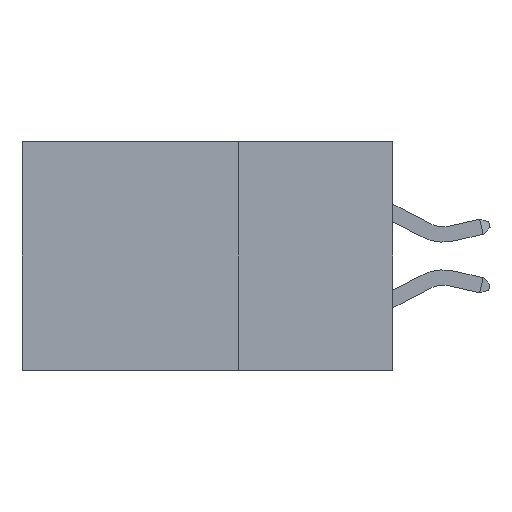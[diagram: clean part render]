
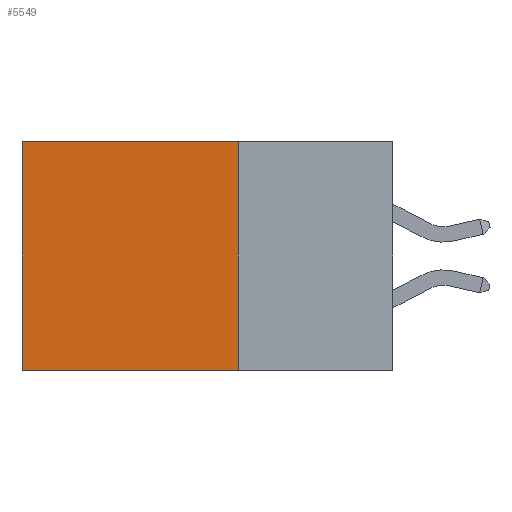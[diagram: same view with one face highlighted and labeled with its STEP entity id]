
A CAD part, left-side view. The second image highlights one B-rep face of the part: STEP entity #5549.
In plain terms, the highlighted planar face has unit normal (-1, 0, 0).
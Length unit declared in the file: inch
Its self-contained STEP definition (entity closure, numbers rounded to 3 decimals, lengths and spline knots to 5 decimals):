
#68 = VERTEX_POINT ( 'NONE', #19197 ) ;
#89 = DIRECTION ( 'NONE',  ( 1., 0., 0. ) ) ;
#135 = CARTESIAN_POINT ( 'NONE',  ( 0.2875, 0.25, 0. ) ) ;
#137 = CARTESIAN_POINT ( 'NONE',  ( 0.2875, 0.6, -0.37 ) ) ;
#147 = ORIENTED_EDGE ( 'NONE', *, *, #17305, .T. ) ;
#314 = DIRECTION ( 'NONE',  ( 0., 0., -1. ) ) ;
#1629 = DIRECTION ( 'NONE',  ( 0., 0., -1. ) ) ;
#2861 = ORIENTED_EDGE ( 'NONE', *, *, #16592, .F. ) ;
#3113 = VERTEX_POINT ( 'NONE', #137 ) ;
#3219 = DIRECTION ( 'NONE',  ( 0., 0., -1. ) ) ;
#3332 = CARTESIAN_POINT ( 'NONE',  ( 0.2875, 0.6, 0. ) ) ;
#3769 = CARTESIAN_POINT ( 'NONE',  ( 0.2875, 0.25, -0.37 ) ) ;
#3929 = PLANE ( 'NONE',  #12392 ) ;
#4336 = VECTOR ( 'NONE', #1629, 39.37008 ) ;
#5140 = DIRECTION ( 'NONE',  ( 0., 1., 0. ) ) ;
#5549 = ADVANCED_FACE ( 'NONE', ( #10672 ), #3929, .F. ) ;
#6506 = VECTOR ( 'NONE', #5140, 39.37008 ) ;
#6512 = VECTOR ( 'NONE', #6896, 39.37008 ) ;
#6896 = DIRECTION ( 'NONE',  ( 0., 1., 0. ) ) ;
#8709 = VECTOR ( 'NONE', #3219, 39.37008 ) ;
#9147 = CARTESIAN_POINT ( 'NONE',  ( 0.2875, 0.25, 0. ) ) ;
#9589 = EDGE_CURVE ( 'NONE', #68, #3113, #10535, .T. ) ;
#9916 = VERTEX_POINT ( 'NONE', #9147 ) ;
#10535 = LINE ( 'NONE', #3769, #6512 ) ;
#10672 = FACE_OUTER_BOUND ( 'NONE', #18408, .T. ) ;
#12073 = CARTESIAN_POINT ( 'NONE',  ( 0.2875, 0.6, 0. ) ) ;
#12135 = ORIENTED_EDGE ( 'NONE', *, *, #17420, .T. ) ;
#12392 = AXIS2_PLACEMENT_3D ( 'NONE', #135, #89, #314 ) ;
#13753 = CARTESIAN_POINT ( 'NONE',  ( 0.2875, 0.25, 0. ) ) ;
#14329 = LINE ( 'NONE', #15424, #6506 ) ;
#15424 = CARTESIAN_POINT ( 'NONE',  ( 0.2875, 0.25, 0. ) ) ;
#15942 = ORIENTED_EDGE ( 'NONE', *, *, #9589, .F. ) ;
#16125 = LINE ( 'NONE', #3332, #4336 ) ;
#16380 = LINE ( 'NONE', #13753, #8709 ) ;
#16592 = EDGE_CURVE ( 'NONE', #9916, #68, #16380, .T. ) ;
#17305 = EDGE_CURVE ( 'NONE', #19078, #3113, #16125, .T. ) ;
#17420 = EDGE_CURVE ( 'NONE', #9916, #19078, #14329, .T. ) ;
#18408 = EDGE_LOOP ( 'NONE', ( #147, #15942, #2861, #12135 ) ) ;
#19078 = VERTEX_POINT ( 'NONE', #12073 ) ;
#19197 = CARTESIAN_POINT ( 'NONE',  ( 0.2875, 0.25, -0.37 ) ) ;
